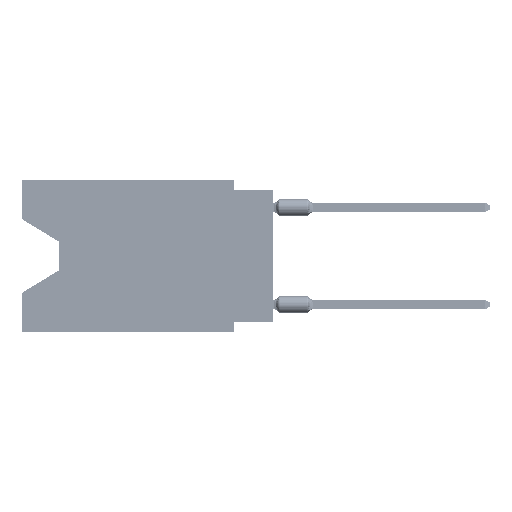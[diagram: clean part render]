
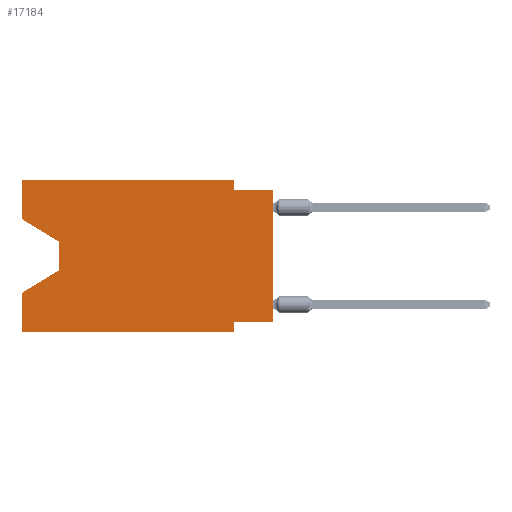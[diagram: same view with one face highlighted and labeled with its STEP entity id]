
A CAD part, left-side view. The second image highlights one B-rep face of the part: STEP entity #17184.
In plain terms, the highlighted planar face has unit normal (-1, 0, 0).
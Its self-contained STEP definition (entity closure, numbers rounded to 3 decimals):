
#54 = VERTEX_POINT ( 'NONE', #35252 ) ;
#555 = ORIENTED_EDGE ( 'NONE', *, *, #41404, .F. ) ;
#698 = CARTESIAN_POINT ( 'NONE',  ( 0., 16.383, 0. ) ) ;
#1109 = DIRECTION ( 'NONE',  ( 0., -1., 0. ) ) ;
#1170 = DIRECTION ( 'NONE',  ( 0., 0., -1. ) ) ;
#1374 = VERTEX_POINT ( 'NONE', #15485 ) ;
#1994 = VERTEX_POINT ( 'NONE', #51351 ) ;
#2821 = VECTOR ( 'NONE', #76006, 1000. ) ;
#4436 = VERTEX_POINT ( 'NONE', #68706 ) ;
#5479 = EDGE_CURVE ( 'NONE', #10410, #1374, #44122, .T. ) ;
#5739 = ORIENTED_EDGE ( 'NONE', *, *, #71432, .T. ) ;
#6034 = DIRECTION ( 'NONE',  ( 0., 0., 1. ) ) ;
#6679 = FACE_OUTER_BOUND ( 'NONE', #9610, .T. ) ;
#7512 = EDGE_CURVE ( 'NONE', #60834, #54, #26324, .T. ) ;
#8668 = ORIENTED_EDGE ( 'NONE', *, *, #22116, .T. ) ;
#9610 = EDGE_LOOP ( 'NONE', ( #63083, #63250, #8668, #52580, #73563, #73699, #74653, #5739, #70878, #68760, #21138, #555 ) ) ;
#10410 = VERTEX_POINT ( 'NONE', #55584 ) ;
#12493 = CARTESIAN_POINT ( 'NONE',  ( 0., 13.97, -5.893 ) ) ;
#12556 = VECTOR ( 'NONE', #41812, 1000. ) ;
#12664 = AXIS2_PLACEMENT_3D ( 'NONE', #74117, #24157, #62299 ) ;
#13357 = LINE ( 'NONE', #57587, #61495 ) ;
#13678 = CARTESIAN_POINT ( 'NONE',  ( 0., 0., -0.635 ) ) ;
#14692 = DIRECTION ( 'NONE',  ( 0., 0., 1. ) ) ;
#15026 = VERTEX_POINT ( 'NONE', #698 ) ;
#15467 = LINE ( 'NONE', #28031, #16802 ) ;
#15485 = CARTESIAN_POINT ( 'NONE',  ( 0., 0., -0.635 ) ) ;
#16136 = CARTESIAN_POINT ( 'NONE',  ( 0., 16.383, -9.906 ) ) ;
#16802 = VECTOR ( 'NONE', #14692, 1000. ) ;
#17075 = CARTESIAN_POINT ( 'NONE',  ( 0., 16.383, -2.546 ) ) ;
#17184 = ADVANCED_FACE ( 'NONE', ( #6679 ), #18860, .F. ) ;
#18126 = DIRECTION ( 'NONE',  ( 0., 0., -1. ) ) ;
#18860 = PLANE ( 'NONE',  #12664 ) ;
#20470 = CARTESIAN_POINT ( 'NONE',  ( 0., 16.383, 0. ) ) ;
#20876 = DIRECTION ( 'NONE',  ( 0., 0., 1. ) ) ;
#21138 = ORIENTED_EDGE ( 'NONE', *, *, #33975, .F. ) ;
#22116 = EDGE_CURVE ( 'NONE', #54, #67688, #68126, .T. ) ;
#23221 = EDGE_CURVE ( 'NONE', #44396, #10410, #24618, .T. ) ;
#24157 = DIRECTION ( 'NONE',  ( 1., 0., 0. ) ) ;
#24216 = VERTEX_POINT ( 'NONE', #64864 ) ;
#24618 = LINE ( 'NONE', #31098, #66326 ) ;
#24766 = LINE ( 'NONE', #17075, #12556 ) ;
#26324 = LINE ( 'NONE', #57972, #63131 ) ;
#26729 = DIRECTION ( 'NONE',  ( 0., 1., 0. ) ) ;
#26943 = DIRECTION ( 'NONE',  ( 0., 0.855, -0.519 ) ) ;
#27877 = LINE ( 'NONE', #72165, #48952 ) ;
#27904 = LINE ( 'NONE', #16136, #70183 ) ;
#28031 = CARTESIAN_POINT ( 'NONE',  ( 0., 0., 0. ) ) ;
#28946 = VECTOR ( 'NONE', #6034, 1000. ) ;
#30661 = VECTOR ( 'NONE', #1109, 1000. ) ;
#31098 = CARTESIAN_POINT ( 'NONE',  ( 0., 2.54, 0. ) ) ;
#33975 = EDGE_CURVE ( 'NONE', #15026, #44396, #27877, .T. ) ;
#35252 = CARTESIAN_POINT ( 'NONE',  ( 0., 13.97, -5.893 ) ) ;
#36470 = CARTESIAN_POINT ( 'NONE',  ( 0., 16.383, 0. ) ) ;
#39356 = LINE ( 'NONE', #36470, #28946 ) ;
#41404 = EDGE_CURVE ( 'NONE', #24216, #15026, #39356, .T. ) ;
#41812 = DIRECTION ( 'NONE',  ( 0., -0.855, -0.519 ) ) ;
#44122 = LINE ( 'NONE', #13678, #30661 ) ;
#44396 = VERTEX_POINT ( 'NONE', #72164 ) ;
#44617 = VERTEX_POINT ( 'NONE', #64742 ) ;
#46025 = LINE ( 'NONE', #20470, #46273 ) ;
#46273 = VECTOR ( 'NONE', #20876, 1000. ) ;
#47435 = EDGE_CURVE ( 'NONE', #24216, #60834, #24766, .T. ) ;
#48952 = VECTOR ( 'NONE', #52646, 1000. ) ;
#50802 = LINE ( 'NONE', #75615, #2821 ) ;
#51351 = CARTESIAN_POINT ( 'NONE',  ( 0., 0., -9.271 ) ) ;
#52580 = ORIENTED_EDGE ( 'NONE', *, *, #59874, .F. ) ;
#52646 = DIRECTION ( 'NONE',  ( 0., -1., 0. ) ) ;
#55584 = CARTESIAN_POINT ( 'NONE',  ( 0., 2.54, -0.635 ) ) ;
#57050 = EDGE_CURVE ( 'NONE', #1994, #44617, #13357, .T. ) ;
#57107 = VECTOR ( 'NONE', #26943, 1000. ) ;
#57587 = CARTESIAN_POINT ( 'NONE',  ( 0., 0., -9.271 ) ) ;
#57972 = CARTESIAN_POINT ( 'NONE',  ( 0., 13.97, -4.013 ) ) ;
#59874 = EDGE_CURVE ( 'NONE', #4436, #67688, #46025, .T. ) ;
#59982 = DIRECTION ( 'NONE',  ( 0., -1., 0. ) ) ;
#60834 = VERTEX_POINT ( 'NONE', #69832 ) ;
#61495 = VECTOR ( 'NONE', #26729, 1000. ) ;
#62299 = DIRECTION ( 'NONE',  ( 0., 0., -1. ) ) ;
#63083 = ORIENTED_EDGE ( 'NONE', *, *, #47435, .T. ) ;
#63131 = VECTOR ( 'NONE', #1170, 1000. ) ;
#63250 = ORIENTED_EDGE ( 'NONE', *, *, #7512, .T. ) ;
#64742 = CARTESIAN_POINT ( 'NONE',  ( 0., 2.54, -9.271 ) ) ;
#64864 = CARTESIAN_POINT ( 'NONE',  ( 0., 16.383, -2.546 ) ) ;
#66326 = VECTOR ( 'NONE', #18126, 1000. ) ;
#66586 = EDGE_CURVE ( 'NONE', #4436, #67590, #27904, .T. ) ;
#67590 = VERTEX_POINT ( 'NONE', #73603 ) ;
#67688 = VERTEX_POINT ( 'NONE', #74010 ) ;
#67795 = EDGE_CURVE ( 'NONE', #44617, #67590, #50802, .T. ) ;
#68126 = LINE ( 'NONE', #12493, #57107 ) ;
#68706 = CARTESIAN_POINT ( 'NONE',  ( 0., 16.383, -9.906 ) ) ;
#68760 = ORIENTED_EDGE ( 'NONE', *, *, #23221, .F. ) ;
#69832 = CARTESIAN_POINT ( 'NONE',  ( 0., 13.97, -4.013 ) ) ;
#70183 = VECTOR ( 'NONE', #59982, 1000. ) ;
#70878 = ORIENTED_EDGE ( 'NONE', *, *, #5479, .F. ) ;
#71432 = EDGE_CURVE ( 'NONE', #1994, #1374, #15467, .T. ) ;
#72164 = CARTESIAN_POINT ( 'NONE',  ( 0., 2.54, 0. ) ) ;
#72165 = CARTESIAN_POINT ( 'NONE',  ( 0., 16.383, 0. ) ) ;
#73563 = ORIENTED_EDGE ( 'NONE', *, *, #66586, .T. ) ;
#73603 = CARTESIAN_POINT ( 'NONE',  ( 0., 2.54, -9.906 ) ) ;
#73699 = ORIENTED_EDGE ( 'NONE', *, *, #67795, .F. ) ;
#74010 = CARTESIAN_POINT ( 'NONE',  ( 0., 16.383, -7.36 ) ) ;
#74117 = CARTESIAN_POINT ( 'NONE',  ( 0., 16.383, 0. ) ) ;
#74653 = ORIENTED_EDGE ( 'NONE', *, *, #57050, .F. ) ;
#75615 = CARTESIAN_POINT ( 'NONE',  ( 0., 2.54, -9.906 ) ) ;
#76006 = DIRECTION ( 'NONE',  ( 0., 0., -1. ) ) ;
